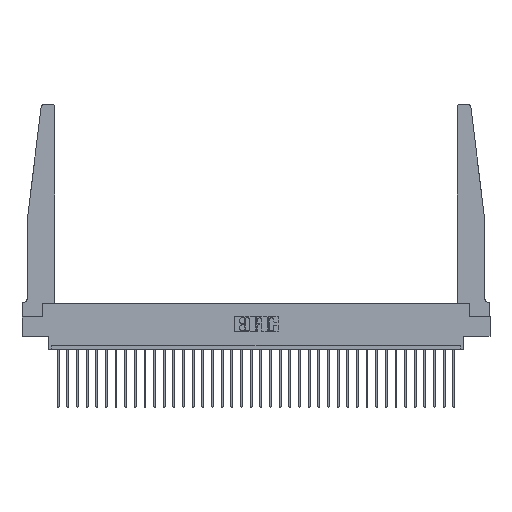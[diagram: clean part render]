
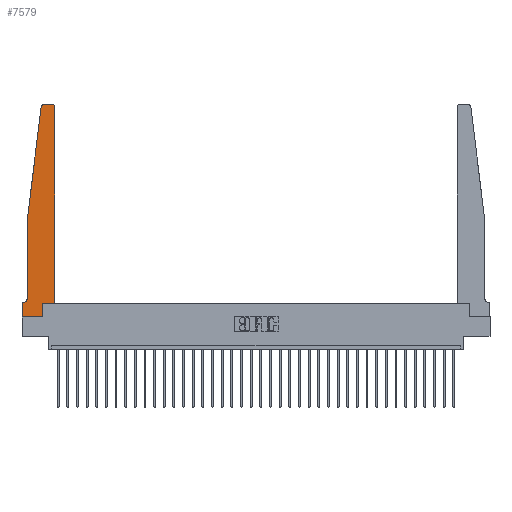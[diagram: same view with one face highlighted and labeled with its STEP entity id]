
A CAD part, top view. The second image highlights one B-rep face of the part: STEP entity #7579.
In plain terms, the highlighted planar face has unit normal (0, 0, 1).
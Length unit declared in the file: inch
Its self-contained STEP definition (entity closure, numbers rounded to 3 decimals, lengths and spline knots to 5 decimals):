
#157 = ORIENTED_EDGE ( 'NONE', *, *, #28470, .T. ) ;
#523 = CARTESIAN_POINT ( 'NONE',  ( 0., 0., 0.37 ) ) ;
#750 = VECTOR ( 'NONE', #1907, 39.37008 ) ;
#1449 = CARTESIAN_POINT ( 'NONE',  ( 0., 0.1875, 0.37 ) ) ;
#1709 = VERTEX_POINT ( 'NONE', #16666 ) ;
#1907 = DIRECTION ( 'NONE',  ( -1., 0., 0. ) ) ;
#1911 = CARTESIAN_POINT ( 'NONE',  ( 0.27653, 2.72, 0.37 ) ) ;
#2836 = EDGE_CURVE ( 'NONE', #18886, #21820, #7754, .T. ) ;
#2855 = FACE_OUTER_BOUND ( 'NONE', #14088, .T. ) ;
#3419 = CARTESIAN_POINT ( 'NONE',  ( 0.425, 0.18, 0.37 ) ) ;
#3911 = LINE ( 'NONE', #25546, #20868 ) ;
#4134 = VERTEX_POINT ( 'NONE', #5225 ) ;
#4207 = AXIS2_PLACEMENT_3D ( 'NONE', #28784, #7289, #21622 ) ;
#5060 = CARTESIAN_POINT ( 'NONE',  ( 0.015, 0.1875, 0.37 ) ) ;
#5201 = EDGE_CURVE ( 'NONE', #19783, #24135, #20568, .T. ) ;
#5225 = CARTESIAN_POINT ( 'NONE',  ( 0., 0., 0.37 ) ) ;
#5608 = EDGE_CURVE ( 'NONE', #1709, #30954, #21156, .T. ) ;
#6302 = CIRCLE ( 'NONE', #12356, 0.03 ) ;
#6715 = ORIENTED_EDGE ( 'NONE', *, *, #2836, .T. ) ;
#7154 = VERTEX_POINT ( 'NONE', #1449 ) ;
#7289 = DIRECTION ( 'NONE',  ( 0., 0., -1. ) ) ;
#7579 = ADVANCED_FACE ( 'NONE', ( #2855 ), #26859, .T. ) ;
#7594 = DIRECTION ( 'NONE',  ( 0., 0., 1. ) ) ;
#7754 = CIRCLE ( 'NONE', #4207, 0.05 ) ;
#7760 = DIRECTION ( 'NONE',  ( 1., 0., 0. ) ) ;
#8098 = EDGE_CURVE ( 'NONE', #7154, #4134, #19126, .T. ) ;
#8455 = DIRECTION ( 'NONE',  ( 1., 0., 0. ) ) ;
#8510 = DIRECTION ( 'NONE',  ( -1., 0., 0. ) ) ;
#8967 = CARTESIAN_POINT ( 'NONE',  ( 0.065, 1.25, 0.37 ) ) ;
#9498 = ORIENTED_EDGE ( 'NONE', *, *, #22697, .T. ) ;
#9522 = DIRECTION ( 'NONE',  ( 1., 0., 0. ) ) ;
#9918 = VERTEX_POINT ( 'NONE', #11329 ) ;
#9921 = VECTOR ( 'NONE', #8455, 39.37008 ) ;
#11032 = EDGE_CURVE ( 'NONE', #21820, #7154, #3911, .T. ) ;
#11286 = ORIENTED_EDGE ( 'NONE', *, *, #14369, .T. ) ;
#11329 = CARTESIAN_POINT ( 'NONE',  ( 0.2605, 0., 0.37 ) ) ;
#11866 = VECTOR ( 'NONE', #23849, 39.37008 ) ;
#12032 = CARTESIAN_POINT ( 'NONE',  ( 0.425, 2.72, 0.37 ) ) ;
#12356 = AXIS2_PLACEMENT_3D ( 'NONE', #1911, #31311, #9522 ) ;
#12949 = DIRECTION ( 'NONE',  ( 0., 1., 0. ) ) ;
#13152 = VECTOR ( 'NONE', #18675, 39.37008 ) ;
#13259 = CARTESIAN_POINT ( 'NONE',  ( 0.065, 1.25, 0.37 ) ) ;
#13580 = ORIENTED_EDGE ( 'NONE', *, *, #5201, .T. ) ;
#13685 = VERTEX_POINT ( 'NONE', #12032 ) ;
#14088 = EDGE_LOOP ( 'NONE', ( #30149, #157, #17357, #9498, #6715, #17580, #19128, #11286, #15448, #13580, #23088, #18793 ) ) ;
#14369 = EDGE_CURVE ( 'NONE', #4134, #9918, #22157, .T. ) ;
#15448 = ORIENTED_EDGE ( 'NONE', *, *, #15805, .T. ) ;
#15698 = VECTOR ( 'NONE', #23162, 39.37008 ) ;
#15805 = EDGE_CURVE ( 'NONE', #9918, #19783, #31027, .T. ) ;
#16666 = CARTESIAN_POINT ( 'NONE',  ( 0.395, 2.75, 0.37 ) ) ;
#17144 = CARTESIAN_POINT ( 'NONE',  ( 0.395, 2.72, 0.37 ) ) ;
#17357 = ORIENTED_EDGE ( 'NONE', *, *, #28385, .T. ) ;
#17580 = ORIENTED_EDGE ( 'NONE', *, *, #11032, .T. ) ;
#17732 = CARTESIAN_POINT ( 'NONE',  ( 0.27653, 2.75, 0.37 ) ) ;
#18197 = CARTESIAN_POINT ( 'NONE',  ( 0.425, 0.18, 0.37 ) ) ;
#18675 = DIRECTION ( 'NONE',  ( 0., -1., 0. ) ) ;
#18793 = ORIENTED_EDGE ( 'NONE', *, *, #28496, .T. ) ;
#18886 = VERTEX_POINT ( 'NONE', #25467 ) ;
#19126 = LINE ( 'NONE', #27914, #15698 ) ;
#19128 = ORIENTED_EDGE ( 'NONE', *, *, #8098, .T. ) ;
#19783 = VERTEX_POINT ( 'NONE', #25826 ) ;
#19923 = DIRECTION ( 'NONE',  ( 1., 0., 0. ) ) ;
#19975 = LINE ( 'NONE', #18197, #23514 ) ;
#20152 = VERTEX_POINT ( 'NONE', #30544 ) ;
#20568 = LINE ( 'NONE', #25653, #9921 ) ;
#20868 = VECTOR ( 'NONE', #8510, 39.37008 ) ;
#21156 = LINE ( 'NONE', #23699, #750 ) ;
#21194 = VECTOR ( 'NONE', #19923, 39.37008 ) ;
#21306 = LINE ( 'NONE', #21628, #11866 ) ;
#21337 = CARTESIAN_POINT ( 'NONE',  ( 0.2605, 0.18, 0.37 ) ) ;
#21622 = DIRECTION ( 'NONE',  ( -1., 0., 0. ) ) ;
#21628 = CARTESIAN_POINT ( 'NONE',  ( 0.065, 1.25, 0.37 ) ) ;
#21655 = DIRECTION ( 'NONE',  ( 0., 1., 0. ) ) ;
#21820 = VERTEX_POINT ( 'NONE', #5060 ) ;
#22091 = DIRECTION ( 'NONE',  ( 1., 0., 0. ) ) ;
#22157 = LINE ( 'NONE', #523, #21194 ) ;
#22239 = CARTESIAN_POINT ( 'NONE',  ( 0., 0.1875, 0.37 ) ) ;
#22697 = EDGE_CURVE ( 'NONE', #31016, #18886, #23773, .T. ) ;
#23088 = ORIENTED_EDGE ( 'NONE', *, *, #25399, .T. ) ;
#23162 = DIRECTION ( 'NONE',  ( 0., -1., 0. ) ) ;
#23514 = VECTOR ( 'NONE', #12949, 39.37008 ) ;
#23699 = CARTESIAN_POINT ( 'NONE',  ( 0.25, 2.75, 0.37 ) ) ;
#23773 = LINE ( 'NONE', #8967, #13152 ) ;
#23849 = DIRECTION ( 'NONE',  ( -0.122, -0.992, 0. ) ) ;
#24088 = CIRCLE ( 'NONE', #30671, 0.03 ) ;
#24135 = VERTEX_POINT ( 'NONE', #3419 ) ;
#25399 = EDGE_CURVE ( 'NONE', #24135, #13685, #19975, .T. ) ;
#25467 = CARTESIAN_POINT ( 'NONE',  ( 0.065, 0.2375, 0.37 ) ) ;
#25546 = CARTESIAN_POINT ( 'NONE',  ( 0.065, 0.1875, 0.37 ) ) ;
#25653 = CARTESIAN_POINT ( 'NONE',  ( 0.425, 0.18, 0.37 ) ) ;
#25679 = AXIS2_PLACEMENT_3D ( 'NONE', #22239, #29559, #7760 ) ;
#25826 = CARTESIAN_POINT ( 'NONE',  ( 0.2605, 0.18, 0.37 ) ) ;
#26859 = PLANE ( 'NONE',  #25679 ) ;
#27914 = CARTESIAN_POINT ( 'NONE',  ( 0., 0., 0.37 ) ) ;
#28385 = EDGE_CURVE ( 'NONE', #20152, #31016, #21306, .T. ) ;
#28470 = EDGE_CURVE ( 'NONE', #30954, #20152, #6302, .T. ) ;
#28496 = EDGE_CURVE ( 'NONE', #13685, #1709, #24088, .T. ) ;
#28784 = CARTESIAN_POINT ( 'NONE',  ( 0.015, 0.2375, 0.37 ) ) ;
#29559 = DIRECTION ( 'NONE',  ( 0., 0., 1. ) ) ;
#30149 = ORIENTED_EDGE ( 'NONE', *, *, #5608, .T. ) ;
#30265 = VECTOR ( 'NONE', #21655, 39.37008 ) ;
#30544 = CARTESIAN_POINT ( 'NONE',  ( 0.24675, 2.72367, 0.37 ) ) ;
#30671 = AXIS2_PLACEMENT_3D ( 'NONE', #17144, #7594, #22091 ) ;
#30954 = VERTEX_POINT ( 'NONE', #17732 ) ;
#31016 = VERTEX_POINT ( 'NONE', #13259 ) ;
#31027 = LINE ( 'NONE', #21337, #30265 ) ;
#31311 = DIRECTION ( 'NONE',  ( 0., 0., 1. ) ) ;
